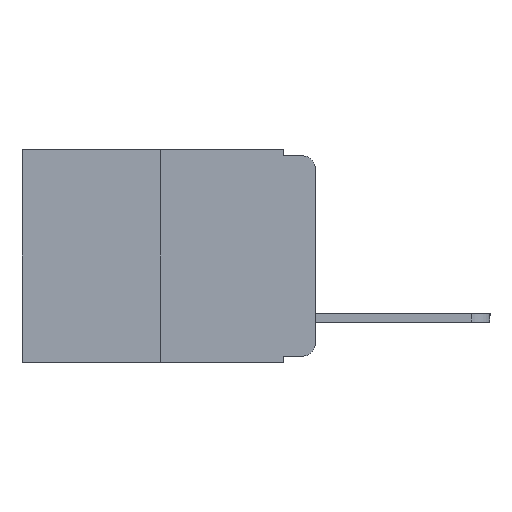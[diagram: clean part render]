
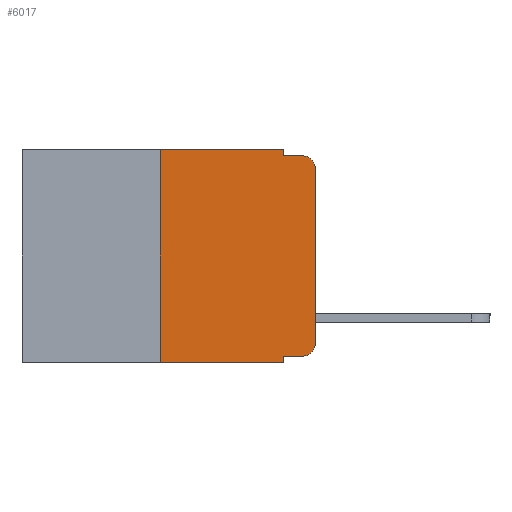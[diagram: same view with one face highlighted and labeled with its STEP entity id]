
A CAD part, left-side view. The second image highlights one B-rep face of the part: STEP entity #6017.
In plain terms, the highlighted planar face has unit normal (-1, 0, 0).
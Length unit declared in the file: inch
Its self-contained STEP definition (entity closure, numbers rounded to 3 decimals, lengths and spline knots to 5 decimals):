
#198 = DIRECTION ( 'NONE',  ( 0., 0., 1. ) ) ;
#254 = DIRECTION ( 'NONE',  ( 0., -1., 0. ) ) ;
#304 = VERTEX_POINT ( 'NONE', #5999 ) ;
#428 = VECTOR ( 'NONE', #6525, 39.37008 ) ;
#489 = VERTEX_POINT ( 'NONE', #9540 ) ;
#528 = VERTEX_POINT ( 'NONE', #4837 ) ;
#613 = DIRECTION ( 'NONE',  ( 0., 0., -1. ) ) ;
#633 = VERTEX_POINT ( 'NONE', #7945 ) ;
#652 = CARTESIAN_POINT ( 'NONE',  ( 0., 0., -0.03 ) ) ;
#667 = CARTESIAN_POINT ( 'NONE',  ( 0., 0.25, 0. ) ) ;
#764 = VECTOR ( 'NONE', #8247, 39.37008 ) ;
#765 = VECTOR ( 'NONE', #3433, 39.37008 ) ;
#932 = ORIENTED_EDGE ( 'NONE', *, *, #10659, .T. ) ;
#996 = ORIENTED_EDGE ( 'NONE', *, *, #11244, .T. ) ;
#1085 = ORIENTED_EDGE ( 'NONE', *, *, #2102, .F. ) ;
#1097 = ORIENTED_EDGE ( 'NONE', *, *, #2209, .T. ) ;
#1200 = ORIENTED_EDGE ( 'NONE', *, *, #3421, .F. ) ;
#1358 = VECTOR ( 'NONE', #8444, 39.37008 ) ;
#1544 = DIRECTION ( 'NONE',  ( 0., -1., 0. ) ) ;
#1607 = VERTEX_POINT ( 'NONE', #667 ) ;
#1609 = CIRCLE ( 'NONE', #10397, 0.02 ) ;
#1617 = ORIENTED_EDGE ( 'NONE', *, *, #10433, .T. ) ;
#1661 = AXIS2_PLACEMENT_3D ( 'NONE', #5470, #11979, #6463 ) ;
#1771 = VECTOR ( 'NONE', #198, 39.37008 ) ;
#2102 = EDGE_CURVE ( 'NONE', #633, #489, #10231, .T. ) ;
#2209 = EDGE_CURVE ( 'NONE', #528, #489, #6615, .T. ) ;
#2788 = FACE_OUTER_BOUND ( 'NONE', #9064, .T. ) ;
#2832 = CARTESIAN_POINT ( 'NONE',  ( 0., 0.051, -0.01 ) ) ;
#3119 = LINE ( 'NONE', #12053, #428 ) ;
#3298 = PLANE ( 'NONE',  #8119 ) ;
#3390 = CARTESIAN_POINT ( 'NONE',  ( 0., 0.051, 0. ) ) ;
#3421 = EDGE_CURVE ( 'NONE', #528, #1607, #10441, .T. ) ;
#3433 = DIRECTION ( 'NONE',  ( 0., 0., -1. ) ) ;
#3452 = LINE ( 'NONE', #3390, #765 ) ;
#3557 = CARTESIAN_POINT ( 'NONE',  ( 0., 0.473, -0.343 ) ) ;
#3628 = EDGE_CURVE ( 'NONE', #1607, #10299, #6397, .T. ) ;
#3774 = VECTOR ( 'NONE', #1544, 39.37008 ) ;
#4069 = EDGE_CURVE ( 'NONE', #10299, #8236, #3452, .T. ) ;
#4253 = CARTESIAN_POINT ( 'NONE',  ( 0., 0.051, -0.01 ) ) ;
#4279 = VERTEX_POINT ( 'NONE', #652 ) ;
#4317 = DIRECTION ( 'NONE',  ( 1., 0., 0. ) ) ;
#4369 = CARTESIAN_POINT ( 'NONE',  ( 0., 0.051, 0. ) ) ;
#4378 = LINE ( 'NONE', #6204, #1771 ) ;
#4687 = ORIENTED_EDGE ( 'NONE', *, *, #6712, .F. ) ;
#4837 = CARTESIAN_POINT ( 'NONE',  ( 0., 0.25, -0.343 ) ) ;
#5221 = ORIENTED_EDGE ( 'NONE', *, *, #4069, .F. ) ;
#5469 = CARTESIAN_POINT ( 'NONE',  ( 0., 0.473, 0. ) ) ;
#5470 = CARTESIAN_POINT ( 'NONE',  ( 0., 0.02, -0.03 ) ) ;
#5983 = ORIENTED_EDGE ( 'NONE', *, *, #3628, .F. ) ;
#5999 = CARTESIAN_POINT ( 'NONE',  ( 0., 0., -0.313 ) ) ;
#6017 = ADVANCED_FACE ( 'NONE', ( #2788 ), #3298, .F. ) ;
#6204 = CARTESIAN_POINT ( 'NONE',  ( 0., 0., 0. ) ) ;
#6247 = ORIENTED_EDGE ( 'NONE', *, *, #7367, .T. ) ;
#6397 = LINE ( 'NONE', #5469, #3774 ) ;
#6463 = DIRECTION ( 'NONE',  ( 0., 0., -1. ) ) ;
#6525 = DIRECTION ( 'NONE',  ( 0., -1., 0. ) ) ;
#6580 = DIRECTION ( 'NONE',  ( -1., 0., 0. ) ) ;
#6615 = LINE ( 'NONE', #3557, #1358 ) ;
#6710 = CARTESIAN_POINT ( 'NONE',  ( 0., 0.02, -0.01 ) ) ;
#6712 = EDGE_CURVE ( 'NONE', #8236, #12044, #10518, .T. ) ;
#7234 = CARTESIAN_POINT ( 'NONE',  ( 0., 0.473, 0. ) ) ;
#7367 = EDGE_CURVE ( 'NONE', #4279, #12044, #8231, .T. ) ;
#7516 = VECTOR ( 'NONE', #254, 39.37008 ) ;
#7945 = CARTESIAN_POINT ( 'NONE',  ( 0., 0.051, -0.333 ) ) ;
#8119 = AXIS2_PLACEMENT_3D ( 'NONE', #7234, #4317, #10934 ) ;
#8152 = VERTEX_POINT ( 'NONE', #8523 ) ;
#8231 = CIRCLE ( 'NONE', #1661, 0.02 ) ;
#8236 = VERTEX_POINT ( 'NONE', #2832 ) ;
#8247 = DIRECTION ( 'NONE',  ( 0., 0., 1. ) ) ;
#8444 = DIRECTION ( 'NONE',  ( 0., -1., 0. ) ) ;
#8523 = CARTESIAN_POINT ( 'NONE',  ( 0., 0.02, -0.333 ) ) ;
#9064 = EDGE_LOOP ( 'NONE', ( #1617, #6247, #4687, #5221, #5983, #1200, #1097, #1085, #996, #932 ) ) ;
#9540 = CARTESIAN_POINT ( 'NONE',  ( 0., 0.051, -0.343 ) ) ;
#10231 = LINE ( 'NONE', #4369, #12385 ) ;
#10299 = VERTEX_POINT ( 'NONE', #11489 ) ;
#10397 = AXIS2_PLACEMENT_3D ( 'NONE', #12109, #6580, #613 ) ;
#10433 = EDGE_CURVE ( 'NONE', #304, #4279, #4378, .T. ) ;
#10441 = LINE ( 'NONE', #11862, #764 ) ;
#10518 = LINE ( 'NONE', #4253, #7516 ) ;
#10659 = EDGE_CURVE ( 'NONE', #8152, #304, #1609, .T. ) ;
#10934 = DIRECTION ( 'NONE',  ( 0., 0., -1. ) ) ;
#10938 = DIRECTION ( 'NONE',  ( 0., 0., -1. ) ) ;
#11244 = EDGE_CURVE ( 'NONE', #633, #8152, #3119, .T. ) ;
#11489 = CARTESIAN_POINT ( 'NONE',  ( 0., 0.051, 0. ) ) ;
#11862 = CARTESIAN_POINT ( 'NONE',  ( 0., 0.25, 0. ) ) ;
#11979 = DIRECTION ( 'NONE',  ( -1., 0., 0. ) ) ;
#12044 = VERTEX_POINT ( 'NONE', #6710 ) ;
#12053 = CARTESIAN_POINT ( 'NONE',  ( 0., 0.051, -0.333 ) ) ;
#12109 = CARTESIAN_POINT ( 'NONE',  ( 0., 0.02, -0.313 ) ) ;
#12385 = VECTOR ( 'NONE', #10938, 39.37008 ) ;
